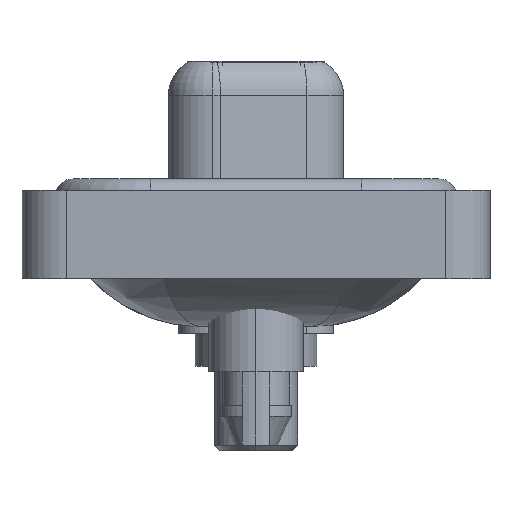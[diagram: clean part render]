
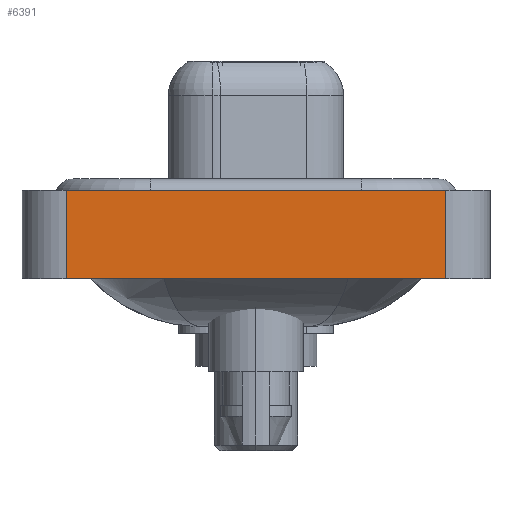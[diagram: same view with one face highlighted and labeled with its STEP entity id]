
A CAD part, left-side view. The second image highlights one B-rep face of the part: STEP entity #6391.
In plain terms, the highlighted planar face has unit normal (-1, 0, 0).
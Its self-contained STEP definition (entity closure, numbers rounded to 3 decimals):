
#265 = VECTOR ( 'NONE', #2935, 1000. ) ;
#384 = CARTESIAN_POINT ( 'NONE',  ( -7.3, -8.55, -3.6 ) ) ;
#2019 = EDGE_CURVE ( 'NONE', #8207, #7893, #14327, .T. ) ;
#2118 = FACE_OUTER_BOUND ( 'NONE', #7994, .T. ) ;
#2935 = DIRECTION ( 'NONE',  ( 0., 0., 1. ) ) ;
#3450 = VECTOR ( 'NONE', #11811, 1000. ) ;
#4397 = LINE ( 'NONE', #9992, #265 ) ;
#4554 = VERTEX_POINT ( 'NONE', #16333 ) ;
#5146 = ORIENTED_EDGE ( 'NONE', *, *, #17140, .F. ) ;
#5315 = DIRECTION ( 'NONE',  ( 0., 0., 1. ) ) ;
#5404 = DIRECTION ( 'NONE',  ( -1., 0., 0. ) ) ;
#5680 = ORIENTED_EDGE ( 'NONE', *, *, #2019, .T. ) ;
#6045 = AXIS2_PLACEMENT_3D ( 'NONE', #11101, #5404, #5315 ) ;
#6391 = ADVANCED_FACE ( 'NONE', ( #2118 ), #7717, .T. ) ;
#6508 = CARTESIAN_POINT ( 'NONE',  ( -7.3, -8.55, -3.6 ) ) ;
#7717 = PLANE ( 'NONE',  #6045 ) ;
#7893 = VERTEX_POINT ( 'NONE', #6508 ) ;
#7994 = EDGE_LOOP ( 'NONE', ( #11735, #16574, #5146, #5680 ) ) ;
#8207 = VERTEX_POINT ( 'NONE', #11445 ) ;
#8351 = CARTESIAN_POINT ( 'NONE',  ( -7.3, 8.55, 0.4 ) ) ;
#9992 = CARTESIAN_POINT ( 'NONE',  ( -7.3, -8.55, -3.6 ) ) ;
#10757 = VECTOR ( 'NONE', #18073, 1000. ) ;
#11016 = VERTEX_POINT ( 'NONE', #8351 ) ;
#11101 = CARTESIAN_POINT ( 'NONE',  ( -7.3, -8.55, -3.6 ) ) ;
#11445 = CARTESIAN_POINT ( 'NONE',  ( -7.3, 8.55, -3.6 ) ) ;
#11735 = ORIENTED_EDGE ( 'NONE', *, *, #12040, .T. ) ;
#11811 = DIRECTION ( 'NONE',  ( 0., 0., 1. ) ) ;
#11899 = CARTESIAN_POINT ( 'NONE',  ( -7.3, 8.55, -3.6 ) ) ;
#12040 = EDGE_CURVE ( 'NONE', #7893, #4554, #4397, .T. ) ;
#13048 = DIRECTION ( 'NONE',  ( 0., -1., 0. ) ) ;
#14327 = LINE ( 'NONE', #384, #17793 ) ;
#14641 = LINE ( 'NONE', #11899, #3450 ) ;
#15300 = LINE ( 'NONE', #17973, #10757 ) ;
#15451 = EDGE_CURVE ( 'NONE', #11016, #4554, #15300, .T. ) ;
#16333 = CARTESIAN_POINT ( 'NONE',  ( -7.3, -8.55, 0.4 ) ) ;
#16574 = ORIENTED_EDGE ( 'NONE', *, *, #15451, .F. ) ;
#17140 = EDGE_CURVE ( 'NONE', #8207, #11016, #14641, .T. ) ;
#17793 = VECTOR ( 'NONE', #13048, 1000. ) ;
#17973 = CARTESIAN_POINT ( 'NONE',  ( -7.3, -8.55, 0.4 ) ) ;
#18073 = DIRECTION ( 'NONE',  ( 0., -1., 0. ) ) ;
